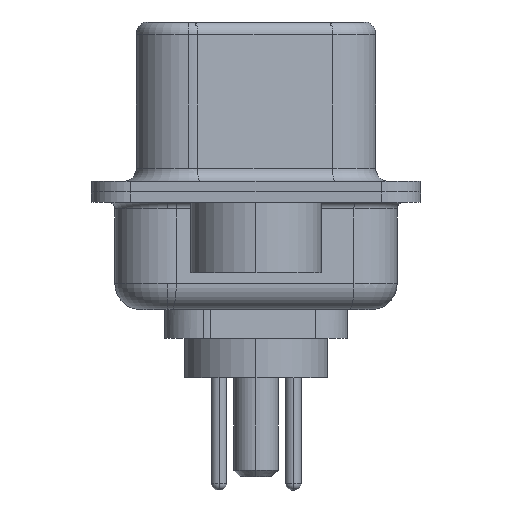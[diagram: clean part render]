
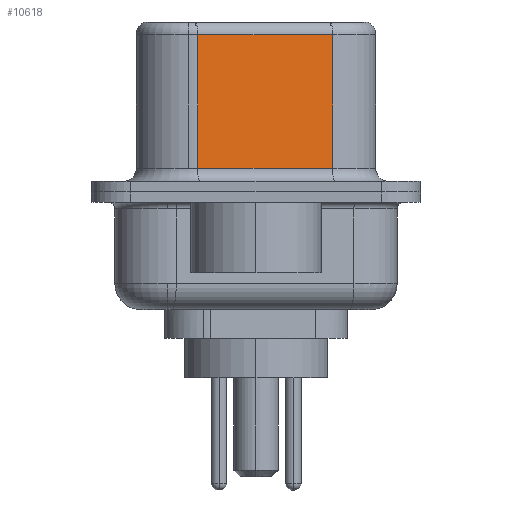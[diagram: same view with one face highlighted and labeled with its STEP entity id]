
A CAD part, left-side view. The second image highlights one B-rep face of the part: STEP entity #10618.
In plain terms, the highlighted planar face has unit normal (-0.985, -0.174, 0).
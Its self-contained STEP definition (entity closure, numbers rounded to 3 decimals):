
#250 = EDGE_CURVE ( 'NONE', #1579, #3760, #2495, .T. ) ;
#278 = VECTOR ( 'NONE', #2502, 1000. ) ;
#798 = CARTESIAN_POINT ( 'NONE',  ( 3.67, 2.233, 6.02 ) ) ;
#976 = VERTEX_POINT ( 'NONE', #18050 ) ;
#1579 = VERTEX_POINT ( 'NONE', #798 ) ;
#2495 = LINE ( 'NONE', #10907, #11774 ) ;
#2502 = DIRECTION ( 'NONE',  ( -0.174, 0.985, 0. ) ) ;
#3760 = VERTEX_POINT ( 'NONE', #16864 ) ;
#3987 = LINE ( 'NONE', #16524, #6083 ) ;
#4759 = PLANE ( 'NONE',  #14920 ) ;
#4878 = VECTOR ( 'NONE', #6546, 1000. ) ;
#5914 = ORIENTED_EDGE ( 'NONE', *, *, #7431, .T. ) ;
#6083 = VECTOR ( 'NONE', #16792, 1000. ) ;
#6426 = CARTESIAN_POINT ( 'NONE',  ( 4.58, -2.927, 0.9 ) ) ;
#6546 = DIRECTION ( 'NONE',  ( 0.174, -0.985, 0. ) ) ;
#6597 = EDGE_CURVE ( 'NONE', #976, #12803, #3987, .T. ) ;
#6722 = LINE ( 'NONE', #18801, #278 ) ;
#7431 = EDGE_CURVE ( 'NONE', #976, #1579, #6722, .T. ) ;
#7712 = DIRECTION ( 'NONE',  ( -0.174, 0.985, 0. ) ) ;
#7851 = LINE ( 'NONE', #14134, #4878 ) ;
#10257 = EDGE_CURVE ( 'NONE', #3760, #12803, #7851, .T. ) ;
#10618 = ADVANCED_FACE ( 'NONE', ( #11806 ), #4759, .F. ) ;
#10907 = CARTESIAN_POINT ( 'NONE',  ( 3.67, 2.233, 6.52 ) ) ;
#11429 = ORIENTED_EDGE ( 'NONE', *, *, #10257, .T. ) ;
#11774 = VECTOR ( 'NONE', #16970, 1000. ) ;
#11793 = DIRECTION ( 'NONE',  ( 0.985, 0.174, 0. ) ) ;
#11806 = FACE_OUTER_BOUND ( 'NONE', #16936, .T. ) ;
#12803 = VERTEX_POINT ( 'NONE', #6426 ) ;
#14134 = CARTESIAN_POINT ( 'NONE',  ( 4.58, -2.927, 0.9 ) ) ;
#14920 = AXIS2_PLACEMENT_3D ( 'NONE', #16633, #11793, #7712 ) ;
#16163 = ORIENTED_EDGE ( 'NONE', *, *, #6597, .F. ) ;
#16524 = CARTESIAN_POINT ( 'NONE',  ( 4.58, -2.927, 6.52 ) ) ;
#16633 = CARTESIAN_POINT ( 'NONE',  ( 4.58, -2.927, 6.52 ) ) ;
#16792 = DIRECTION ( 'NONE',  ( 0., 0., -1. ) ) ;
#16864 = CARTESIAN_POINT ( 'NONE',  ( 3.67, 2.233, 0.9 ) ) ;
#16936 = EDGE_LOOP ( 'NONE', ( #16163, #5914, #18980, #11429 ) ) ;
#16970 = DIRECTION ( 'NONE',  ( 0., 0., -1. ) ) ;
#18050 = CARTESIAN_POINT ( 'NONE',  ( 4.58, -2.927, 6.02 ) ) ;
#18801 = CARTESIAN_POINT ( 'NONE',  ( 4.58, -2.927, 6.02 ) ) ;
#18980 = ORIENTED_EDGE ( 'NONE', *, *, #250, .T. ) ;
